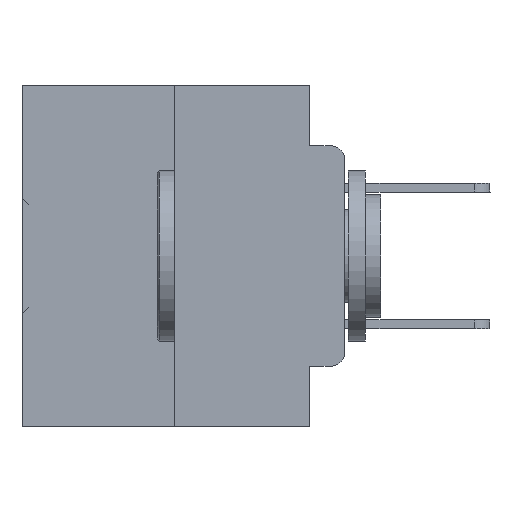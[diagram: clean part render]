
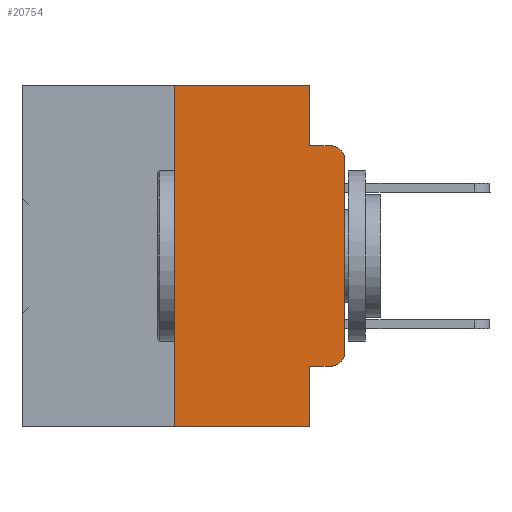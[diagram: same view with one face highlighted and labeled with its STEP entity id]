
A CAD part, left-side view. The second image highlights one B-rep face of the part: STEP entity #20754.
In plain terms, the highlighted planar face has unit normal (-1, 0, 0).
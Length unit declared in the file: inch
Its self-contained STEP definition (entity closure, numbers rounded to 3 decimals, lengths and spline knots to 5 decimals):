
#662 = CARTESIAN_POINT ( 'NONE',  ( 0., 0.02, -0.1085 ) ) ;
#1098 = ORIENTED_EDGE ( 'NONE', *, *, #29253, .T. ) ;
#1192 = DIRECTION ( 'NONE',  ( 0., -1., 0. ) ) ;
#1287 = VECTOR ( 'NONE', #20770, 39.37008 ) ;
#1446 = EDGE_CURVE ( 'NONE', #18270, #6366, #33796, .T. ) ;
#1787 = DIRECTION ( 'NONE',  ( 0., 0., -1. ) ) ;
#3296 = EDGE_CURVE ( 'NONE', #9411, #20432, #33383, .T. ) ;
#3539 = FACE_OUTER_BOUND ( 'NONE', #3900, .T. ) ;
#3829 = CARTESIAN_POINT ( 'NONE',  ( 0., 0.051, -0.5 ) ) ;
#3900 = EDGE_LOOP ( 'NONE', ( #35823, #35137, #9766, #28632, #8200, #17424, #19458, #8239, #1098, #34232 ) ) ;
#4060 = CARTESIAN_POINT ( 'NONE',  ( 0., 0.051, -0.4115 ) ) ;
#4169 = CARTESIAN_POINT ( 'NONE',  ( 0., 0.051, 0. ) ) ;
#5211 = EDGE_CURVE ( 'NONE', #36684, #30407, #35062, .T. ) ;
#6366 = VERTEX_POINT ( 'NONE', #24429 ) ;
#6580 = CIRCLE ( 'NONE', #10860, 0.02 ) ;
#6952 = CARTESIAN_POINT ( 'NONE',  ( 0., 0., -0.1085 ) ) ;
#7189 = DIRECTION ( 'NONE',  ( 0., 0., 1. ) ) ;
#7476 = LINE ( 'NONE', #4060, #28807 ) ;
#7967 = VERTEX_POINT ( 'NONE', #3829 ) ;
#8200 = ORIENTED_EDGE ( 'NONE', *, *, #1446, .F. ) ;
#8239 = ORIENTED_EDGE ( 'NONE', *, *, #9256, .F. ) ;
#8548 = CARTESIAN_POINT ( 'NONE',  ( 0., 0.02, -0.3915 ) ) ;
#8652 = EDGE_CURVE ( 'NONE', #6366, #9411, #30621, .T. ) ;
#8721 = VERTEX_POINT ( 'NONE', #6952 ) ;
#8774 = EDGE_CURVE ( 'NONE', #8721, #20432, #6580, .T. ) ;
#9256 = EDGE_CURVE ( 'NONE', #16282, #7967, #11891, .T. ) ;
#9283 = LINE ( 'NONE', #15385, #37537 ) ;
#9411 = VERTEX_POINT ( 'NONE', #31286 ) ;
#9766 = ORIENTED_EDGE ( 'NONE', *, *, #3296, .F. ) ;
#9821 = CARTESIAN_POINT ( 'NONE',  ( 0., 0.473, 0. ) ) ;
#10137 = LINE ( 'NONE', #21767, #30871 ) ;
#10860 = AXIS2_PLACEMENT_3D ( 'NONE', #662, #29609, #23916 ) ;
#11237 = VECTOR ( 'NONE', #33191, 39.37008 ) ;
#11370 = AXIS2_PLACEMENT_3D ( 'NONE', #8548, #14829, #32522 ) ;
#11475 = VECTOR ( 'NONE', #1787, 39.37008 ) ;
#11681 = CARTESIAN_POINT ( 'NONE',  ( 0., 0.051, -0.4115 ) ) ;
#11891 = LINE ( 'NONE', #13207, #11475 ) ;
#12672 = DIRECTION ( 'NONE',  ( 0., -1., 0. ) ) ;
#13207 = CARTESIAN_POINT ( 'NONE',  ( 0., 0.051, 0. ) ) ;
#14829 = DIRECTION ( 'NONE',  ( -1., 0., 0. ) ) ;
#15154 = PLANE ( 'NONE',  #26161 ) ;
#15385 = CARTESIAN_POINT ( 'NONE',  ( 0., 0., 0. ) ) ;
#15927 = EDGE_CURVE ( 'NONE', #30407, #8721, #9283, .T. ) ;
#16282 = VERTEX_POINT ( 'NONE', #11681 ) ;
#17424 = ORIENTED_EDGE ( 'NONE', *, *, #21455, .F. ) ;
#18155 = EDGE_CURVE ( 'NONE', #18958, #7967, #10137, .T. ) ;
#18270 = VERTEX_POINT ( 'NONE', #19099 ) ;
#18464 = CARTESIAN_POINT ( 'NONE',  ( 0., 0.25, 0. ) ) ;
#18521 = DIRECTION ( 'NONE',  ( 0., -1., 0. ) ) ;
#18958 = VERTEX_POINT ( 'NONE', #26426 ) ;
#19099 = CARTESIAN_POINT ( 'NONE',  ( 0., 0.25, 0. ) ) ;
#19458 = ORIENTED_EDGE ( 'NONE', *, *, #18155, .T. ) ;
#20432 = VERTEX_POINT ( 'NONE', #30995 ) ;
#20754 = ADVANCED_FACE ( 'NONE', ( #3539 ), #15154, .F. ) ;
#20770 = DIRECTION ( 'NONE',  ( 0., 0., 1. ) ) ;
#21455 = EDGE_CURVE ( 'NONE', #18958, #18270, #30063, .T. ) ;
#21596 = CARTESIAN_POINT ( 'NONE',  ( 0., 0.051, -0.0885 ) ) ;
#21767 = CARTESIAN_POINT ( 'NONE',  ( 0., 0.473, -0.5 ) ) ;
#23916 = DIRECTION ( 'NONE',  ( 0., 0., -1. ) ) ;
#23925 = DIRECTION ( 'NONE',  ( 0., 0., -1. ) ) ;
#24429 = CARTESIAN_POINT ( 'NONE',  ( 0., 0.051, 0. ) ) ;
#26161 = AXIS2_PLACEMENT_3D ( 'NONE', #27134, #30176, #23925 ) ;
#26426 = CARTESIAN_POINT ( 'NONE',  ( 0., 0.25, -0.5 ) ) ;
#27134 = CARTESIAN_POINT ( 'NONE',  ( 0., 0.473, 0. ) ) ;
#28632 = ORIENTED_EDGE ( 'NONE', *, *, #8652, .F. ) ;
#28807 = VECTOR ( 'NONE', #1192, 39.37008 ) ;
#29253 = EDGE_CURVE ( 'NONE', #16282, #36684, #7476, .T. ) ;
#29609 = DIRECTION ( 'NONE',  ( -1., 0., 0. ) ) ;
#29797 = CARTESIAN_POINT ( 'NONE',  ( 0., 0., -0.3915 ) ) ;
#30063 = LINE ( 'NONE', #18464, #1287 ) ;
#30176 = DIRECTION ( 'NONE',  ( 1., 0., 0. ) ) ;
#30203 = VECTOR ( 'NONE', #12672, 39.37008 ) ;
#30378 = CARTESIAN_POINT ( 'NONE',  ( 0., 0.02, -0.4115 ) ) ;
#30407 = VERTEX_POINT ( 'NONE', #29797 ) ;
#30431 = DIRECTION ( 'NONE',  ( 0., 0., -1. ) ) ;
#30621 = LINE ( 'NONE', #4169, #35165 ) ;
#30871 = VECTOR ( 'NONE', #18521, 39.37008 ) ;
#30995 = CARTESIAN_POINT ( 'NONE',  ( 0., 0.02, -0.0885 ) ) ;
#31286 = CARTESIAN_POINT ( 'NONE',  ( 0., 0.051, -0.0885 ) ) ;
#32522 = DIRECTION ( 'NONE',  ( 0., 0., -1. ) ) ;
#33191 = DIRECTION ( 'NONE',  ( 0., -1., 0. ) ) ;
#33383 = LINE ( 'NONE', #21596, #11237 ) ;
#33796 = LINE ( 'NONE', #9821, #30203 ) ;
#34232 = ORIENTED_EDGE ( 'NONE', *, *, #5211, .T. ) ;
#35062 = CIRCLE ( 'NONE', #11370, 0.02 ) ;
#35137 = ORIENTED_EDGE ( 'NONE', *, *, #8774, .T. ) ;
#35165 = VECTOR ( 'NONE', #30431, 39.37008 ) ;
#35823 = ORIENTED_EDGE ( 'NONE', *, *, #15927, .T. ) ;
#36684 = VERTEX_POINT ( 'NONE', #30378 ) ;
#37537 = VECTOR ( 'NONE', #7189, 39.37008 ) ;
